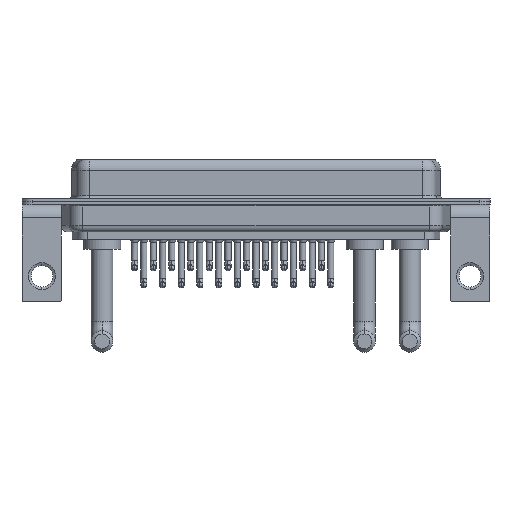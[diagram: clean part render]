
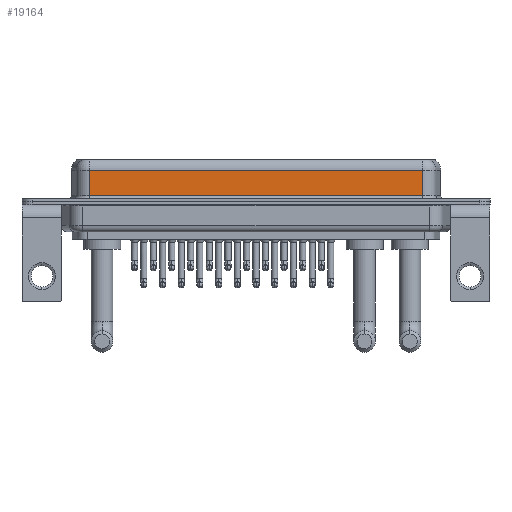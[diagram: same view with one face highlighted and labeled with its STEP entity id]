
A CAD part, front view. The second image highlights one B-rep face of the part: STEP entity #19164.
In plain terms, the highlighted planar face has unit normal (0, -1, 0).
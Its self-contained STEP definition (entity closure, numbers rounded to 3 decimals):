
#1401 = DIRECTION ( 'NONE',  ( 0., 0., -1. ) ) ;
#1490 = CARTESIAN_POINT ( 'NONE',  ( 7.038, -3.95, 4.65 ) ) ;
#1716 = ORIENTED_EDGE ( 'NONE', *, *, #8348, .T. ) ;
#3991 = CARTESIAN_POINT ( 'NONE',  ( 56.462, -3.95, 4.65 ) ) ;
#4240 = CARTESIAN_POINT ( 'NONE',  ( 56.462, -3.95, 6.4 ) ) ;
#5987 = FACE_OUTER_BOUND ( 'NONE', #9105, .T. ) ;
#6676 = CARTESIAN_POINT ( 'NONE',  ( 56.462, -3.95, 0.9 ) ) ;
#7950 = VERTEX_POINT ( 'NONE', #22171 ) ;
#8348 = EDGE_CURVE ( 'NONE', #7950, #11227, #10758, .T. ) ;
#9105 = EDGE_LOOP ( 'NONE', ( #15909, #12523, #19617, #1716 ) ) ;
#9398 = DIRECTION ( 'NONE',  ( -1., 0., 0. ) ) ;
#9872 = EDGE_CURVE ( 'NONE', #16783, #11227, #16889, .T. ) ;
#10758 = LINE ( 'NONE', #6676, #24441 ) ;
#10824 = CARTESIAN_POINT ( 'NONE',  ( 7.038, -3.95, 6.4 ) ) ;
#11017 = AXIS2_PLACEMENT_3D ( 'NONE', #4240, #21302, #24540 ) ;
#11227 = VERTEX_POINT ( 'NONE', #16687 ) ;
#11317 = EDGE_CURVE ( 'NONE', #11754, #7950, #20552, .T. ) ;
#11754 = VERTEX_POINT ( 'NONE', #1490 ) ;
#12489 = DIRECTION ( 'NONE',  ( 1., 0., 0. ) ) ;
#12523 = ORIENTED_EDGE ( 'NONE', *, *, #15204, .T. ) ;
#13106 = LINE ( 'NONE', #20491, #16877 ) ;
#15204 = EDGE_CURVE ( 'NONE', #16783, #11754, #13106, .T. ) ;
#15909 = ORIENTED_EDGE ( 'NONE', *, *, #9872, .F. ) ;
#16687 = CARTESIAN_POINT ( 'NONE',  ( 56.462, -3.95, 0.9 ) ) ;
#16783 = VERTEX_POINT ( 'NONE', #3991 ) ;
#16877 = VECTOR ( 'NONE', #9398, 1000. ) ;
#16889 = LINE ( 'NONE', #18522, #19678 ) ;
#18149 = VECTOR ( 'NONE', #1401, 1000. ) ;
#18522 = CARTESIAN_POINT ( 'NONE',  ( 56.462, -3.95, 6.4 ) ) ;
#19164 = ADVANCED_FACE ( 'NONE', ( #5987 ), #21065, .F. ) ;
#19617 = ORIENTED_EDGE ( 'NONE', *, *, #11317, .T. ) ;
#19678 = VECTOR ( 'NONE', #22633, 1000. ) ;
#20491 = CARTESIAN_POINT ( 'NONE',  ( 56.462, -3.95, 4.65 ) ) ;
#20552 = LINE ( 'NONE', #10824, #18149 ) ;
#21065 = PLANE ( 'NONE',  #11017 ) ;
#21302 = DIRECTION ( 'NONE',  ( 0., 1., 0. ) ) ;
#22171 = CARTESIAN_POINT ( 'NONE',  ( 7.038, -3.95, 0.9 ) ) ;
#22633 = DIRECTION ( 'NONE',  ( 0., 0., -1. ) ) ;
#24441 = VECTOR ( 'NONE', #12489, 1000. ) ;
#24540 = DIRECTION ( 'NONE',  ( 0., 0., 1. ) ) ;
